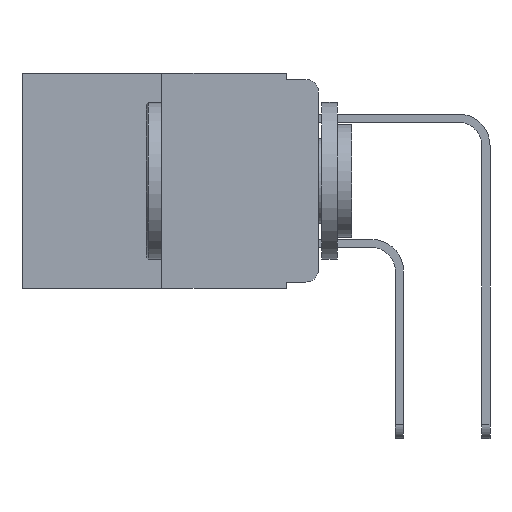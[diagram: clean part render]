
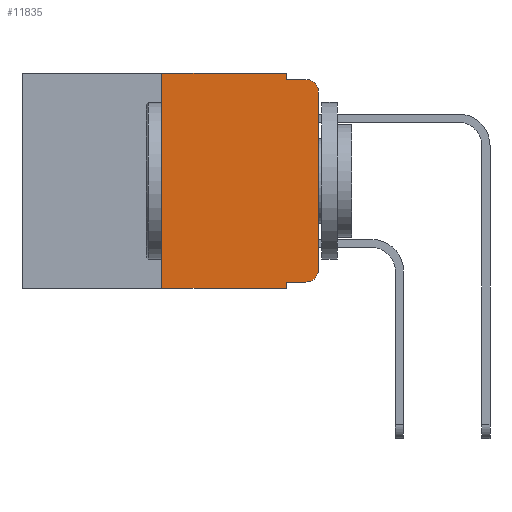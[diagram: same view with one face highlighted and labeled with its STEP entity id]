
A CAD part, left-side view. The second image highlights one B-rep face of the part: STEP entity #11835.
In plain terms, the highlighted planar face has unit normal (-1, 0, 0).
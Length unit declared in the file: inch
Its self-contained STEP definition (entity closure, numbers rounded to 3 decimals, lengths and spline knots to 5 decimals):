
#1009 = EDGE_CURVE ( 'NONE', #1555, #3471, #7416, .T. ) ;
#1111 = VERTEX_POINT ( 'NONE', #14033 ) ;
#1156 = LINE ( 'NONE', #5966, #13994 ) ;
#1295 = ORIENTED_EDGE ( 'NONE', *, *, #9894, .T. ) ;
#1326 = DIRECTION ( 'NONE',  ( 0., -1., 0. ) ) ;
#1333 = ORIENTED_EDGE ( 'NONE', *, *, #11477, .F. ) ;
#1555 = VERTEX_POINT ( 'NONE', #3281 ) ;
#1864 = LINE ( 'NONE', #4301, #11172 ) ;
#2109 = AXIS2_PLACEMENT_3D ( 'NONE', #3107, #12632, #5712 ) ;
#2502 = DIRECTION ( 'NONE',  ( 0., 0., -1. ) ) ;
#3107 = CARTESIAN_POINT ( 'NONE',  ( 0., 0.473, 0. ) ) ;
#3281 = CARTESIAN_POINT ( 'NONE',  ( 0., 0.25, -0.343 ) ) ;
#3335 = DIRECTION ( 'NONE',  ( 0., 0., -1. ) ) ;
#3471 = VERTEX_POINT ( 'NONE', #12309 ) ;
#3740 = FACE_OUTER_BOUND ( 'NONE', #5182, .T. ) ;
#3973 = VERTEX_POINT ( 'NONE', #5634 ) ;
#4301 = CARTESIAN_POINT ( 'NONE',  ( 0., 0.051, -0.333 ) ) ;
#4390 = LINE ( 'NONE', #10441, #4775 ) ;
#4775 = VECTOR ( 'NONE', #3335, 39.37008 ) ;
#4848 = CARTESIAN_POINT ( 'NONE',  ( 0., 0.473, -0.343 ) ) ;
#5182 = EDGE_LOOP ( 'NONE', ( #8899, #13836, #12079, #10983, #13341, #1333, #6362, #6105, #1295, #13452 ) ) ;
#5556 = DIRECTION ( 'NONE',  ( 0., -1., 0. ) ) ;
#5627 = DIRECTION ( 'NONE',  ( -1., 0., 0. ) ) ;
#5634 = CARTESIAN_POINT ( 'NONE',  ( 0., 0.051, 0. ) ) ;
#5712 = DIRECTION ( 'NONE',  ( 0., 0., -1. ) ) ;
#5812 = CIRCLE ( 'NONE', #10598, 0.02 ) ;
#5860 = LINE ( 'NONE', #9666, #8522 ) ;
#5966 = CARTESIAN_POINT ( 'NONE',  ( 0., 0.473, 0. ) ) ;
#6105 = ORIENTED_EDGE ( 'NONE', *, *, #10670, .F. ) ;
#6180 = DIRECTION ( 'NONE',  ( 0., 0., 1. ) ) ;
#6362 = ORIENTED_EDGE ( 'NONE', *, *, #1009, .T. ) ;
#6432 = VECTOR ( 'NONE', #6180, 39.37008 ) ;
#6754 = CARTESIAN_POINT ( 'NONE',  ( 0., 0.25, 0. ) ) ;
#6974 = CARTESIAN_POINT ( 'NONE',  ( 0., 0., -0.313 ) ) ;
#7416 = LINE ( 'NONE', #4848, #10856 ) ;
#7694 = CARTESIAN_POINT ( 'NONE',  ( 0., 0.02, -0.03 ) ) ;
#7761 = AXIS2_PLACEMENT_3D ( 'NONE', #7694, #15724, #8841 ) ;
#8009 = VECTOR ( 'NONE', #2502, 39.37008 ) ;
#8174 = VERTEX_POINT ( 'NONE', #9536 ) ;
#8522 = VECTOR ( 'NONE', #1326, 39.37008 ) ;
#8841 = DIRECTION ( 'NONE',  ( 0., 0., -1. ) ) ;
#8895 = VERTEX_POINT ( 'NONE', #11995 ) ;
#8899 = ORIENTED_EDGE ( 'NONE', *, *, #14557, .T. ) ;
#8998 = CARTESIAN_POINT ( 'NONE',  ( 0., 0.051, -0.333 ) ) ;
#9113 = VERTEX_POINT ( 'NONE', #10079 ) ;
#9135 = EDGE_CURVE ( 'NONE', #8895, #14355, #5812, .T. ) ;
#9536 = CARTESIAN_POINT ( 'NONE',  ( 0., 0.02, -0.01 ) ) ;
#9666 = CARTESIAN_POINT ( 'NONE',  ( 0., 0.051, -0.01 ) ) ;
#9758 = DIRECTION ( 'NONE',  ( 0., 0., 1. ) ) ;
#9894 = EDGE_CURVE ( 'NONE', #14899, #8895, #1864, .T. ) ;
#10079 = CARTESIAN_POINT ( 'NONE',  ( 0., 0.051, -0.01 ) ) ;
#10265 = PLANE ( 'NONE',  #2109 ) ;
#10441 = CARTESIAN_POINT ( 'NONE',  ( 0., 0.051, 0. ) ) ;
#10598 = AXIS2_PLACEMENT_3D ( 'NONE', #12544, #5627, #13669 ) ;
#10670 = EDGE_CURVE ( 'NONE', #14899, #3471, #4390, .T. ) ;
#10856 = VECTOR ( 'NONE', #12987, 39.37008 ) ;
#10983 = ORIENTED_EDGE ( 'NONE', *, *, #12271, .F. ) ;
#11098 = LINE ( 'NONE', #14399, #8009 ) ;
#11172 = VECTOR ( 'NONE', #5556, 39.37008 ) ;
#11477 = EDGE_CURVE ( 'NONE', #1555, #15662, #15580, .T. ) ;
#11835 = ADVANCED_FACE ( 'NONE', ( #3740 ), #10265, .F. ) ;
#11922 = CARTESIAN_POINT ( 'NONE',  ( 0., 0., 0. ) ) ;
#11995 = CARTESIAN_POINT ( 'NONE',  ( 0., 0.02, -0.333 ) ) ;
#12061 = CIRCLE ( 'NONE', #7761, 0.02 ) ;
#12079 = ORIENTED_EDGE ( 'NONE', *, *, #13036, .F. ) ;
#12223 = LINE ( 'NONE', #11922, #6432 ) ;
#12271 = EDGE_CURVE ( 'NONE', #3973, #9113, #11098, .T. ) ;
#12309 = CARTESIAN_POINT ( 'NONE',  ( 0., 0.051, -0.343 ) ) ;
#12544 = CARTESIAN_POINT ( 'NONE',  ( 0., 0.02, -0.313 ) ) ;
#12590 = VECTOR ( 'NONE', #9758, 39.37008 ) ;
#12632 = DIRECTION ( 'NONE',  ( 1., 0., 0. ) ) ;
#12987 = DIRECTION ( 'NONE',  ( 0., -1., 0. ) ) ;
#13036 = EDGE_CURVE ( 'NONE', #9113, #8174, #5860, .T. ) ;
#13341 = ORIENTED_EDGE ( 'NONE', *, *, #14459, .F. ) ;
#13452 = ORIENTED_EDGE ( 'NONE', *, *, #9135, .T. ) ;
#13669 = DIRECTION ( 'NONE',  ( 0., 0., -1. ) ) ;
#13777 = EDGE_CURVE ( 'NONE', #1111, #8174, #12061, .T. ) ;
#13836 = ORIENTED_EDGE ( 'NONE', *, *, #13777, .T. ) ;
#13994 = VECTOR ( 'NONE', #14014, 39.37008 ) ;
#14014 = DIRECTION ( 'NONE',  ( 0., -1., 0. ) ) ;
#14033 = CARTESIAN_POINT ( 'NONE',  ( 0., 0., -0.03 ) ) ;
#14355 = VERTEX_POINT ( 'NONE', #6974 ) ;
#14369 = CARTESIAN_POINT ( 'NONE',  ( 0., 0.25, 0. ) ) ;
#14399 = CARTESIAN_POINT ( 'NONE',  ( 0., 0.051, 0. ) ) ;
#14459 = EDGE_CURVE ( 'NONE', #15662, #3973, #1156, .T. ) ;
#14557 = EDGE_CURVE ( 'NONE', #14355, #1111, #12223, .T. ) ;
#14899 = VERTEX_POINT ( 'NONE', #8998 ) ;
#15580 = LINE ( 'NONE', #14369, #12590 ) ;
#15662 = VERTEX_POINT ( 'NONE', #6754 ) ;
#15724 = DIRECTION ( 'NONE',  ( -1., 0., 0. ) ) ;
